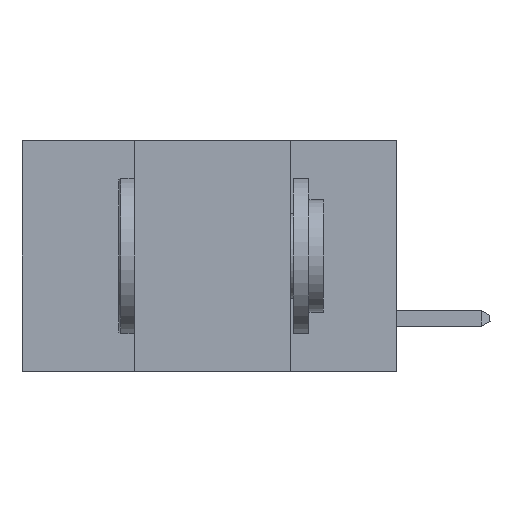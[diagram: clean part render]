
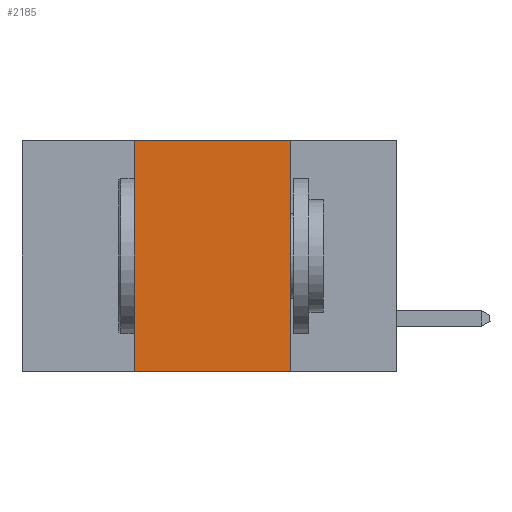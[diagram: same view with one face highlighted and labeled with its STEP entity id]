
A CAD part, left-side view. The second image highlights one B-rep face of the part: STEP entity #2185.
In plain terms, the highlighted planar face has unit normal (-1, 0, 0).
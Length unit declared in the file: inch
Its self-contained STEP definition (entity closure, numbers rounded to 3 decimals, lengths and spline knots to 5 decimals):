
#54 = ORIENTED_EDGE ( 'NONE', *, *, #13213, .F. ) ;
#443 = CARTESIAN_POINT ( 'NONE',  ( 0., 0.42, 0. ) ) ;
#1261 = LINE ( 'NONE', #6255, #9431 ) ;
#1271 = DIRECTION ( 'NONE',  ( 0., 0., -1. ) ) ;
#1333 = DIRECTION ( 'NONE',  ( 1., 0., 0. ) ) ;
#1716 = DIRECTION ( 'NONE',  ( 0., 0., 1. ) ) ;
#2122 = EDGE_CURVE ( 'NONE', #4431, #5790, #4651, .T. ) ;
#2185 = ADVANCED_FACE ( 'NONE', ( #14157 ), #11079, .F. ) ;
#3002 = EDGE_CURVE ( 'NONE', #6412, #4431, #1261, .T. ) ;
#4413 = DIRECTION ( 'NONE',  ( 0., -1., 0. ) ) ;
#4431 = VERTEX_POINT ( 'NONE', #13865 ) ;
#4651 = LINE ( 'NONE', #8269, #9633 ) ;
#5617 = VECTOR ( 'NONE', #1716, 39.37008 ) ;
#5790 = VERTEX_POINT ( 'NONE', #8762 ) ;
#6223 = DIRECTION ( 'NONE',  ( 0., -1., 0. ) ) ;
#6255 = CARTESIAN_POINT ( 'NONE',  ( 0., 0.6, 0. ) ) ;
#6278 = ORIENTED_EDGE ( 'NONE', *, *, #13469, .T. ) ;
#6412 = VERTEX_POINT ( 'NONE', #12534 ) ;
#6426 = VERTEX_POINT ( 'NONE', #11554 ) ;
#7222 = AXIS2_PLACEMENT_3D ( 'NONE', #8302, #1333, #1271 ) ;
#7296 = EDGE_LOOP ( 'NONE', ( #11244, #8779, #54, #6278 ) ) ;
#7827 = DIRECTION ( 'NONE',  ( 0., 0., -1. ) ) ;
#8269 = CARTESIAN_POINT ( 'NONE',  ( 0., 0.17, 0. ) ) ;
#8302 = CARTESIAN_POINT ( 'NONE',  ( 0., 0.6, 0. ) ) ;
#8762 = CARTESIAN_POINT ( 'NONE',  ( 0., 0.17, -0.37 ) ) ;
#8779 = ORIENTED_EDGE ( 'NONE', *, *, #3002, .F. ) ;
#9431 = VECTOR ( 'NONE', #6223, 39.37008 ) ;
#9633 = VECTOR ( 'NONE', #7827, 39.37008 ) ;
#10753 = CARTESIAN_POINT ( 'NONE',  ( 0., 0.6, -0.37 ) ) ;
#11079 = PLANE ( 'NONE',  #7222 ) ;
#11244 = ORIENTED_EDGE ( 'NONE', *, *, #2122, .F. ) ;
#11285 = LINE ( 'NONE', #443, #5617 ) ;
#11554 = CARTESIAN_POINT ( 'NONE',  ( 0., 0.42, -0.37 ) ) ;
#11777 = VECTOR ( 'NONE', #4413, 39.37008 ) ;
#12089 = LINE ( 'NONE', #10753, #11777 ) ;
#12534 = CARTESIAN_POINT ( 'NONE',  ( 0., 0.42, 0. ) ) ;
#13213 = EDGE_CURVE ( 'NONE', #6426, #6412, #11285, .T. ) ;
#13469 = EDGE_CURVE ( 'NONE', #6426, #5790, #12089, .T. ) ;
#13865 = CARTESIAN_POINT ( 'NONE',  ( 0., 0.17, 0. ) ) ;
#14157 = FACE_OUTER_BOUND ( 'NONE', #7296, .T. ) ;
